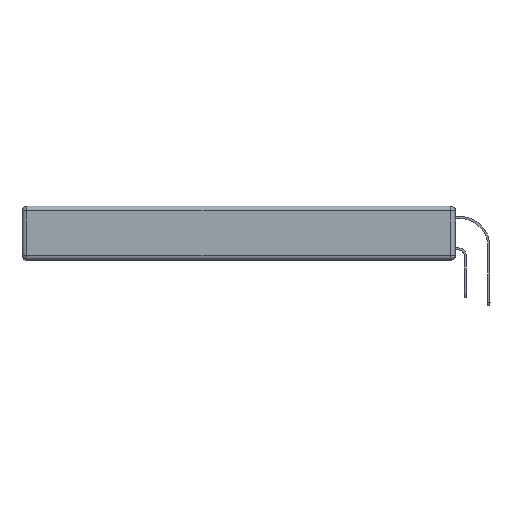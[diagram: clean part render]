
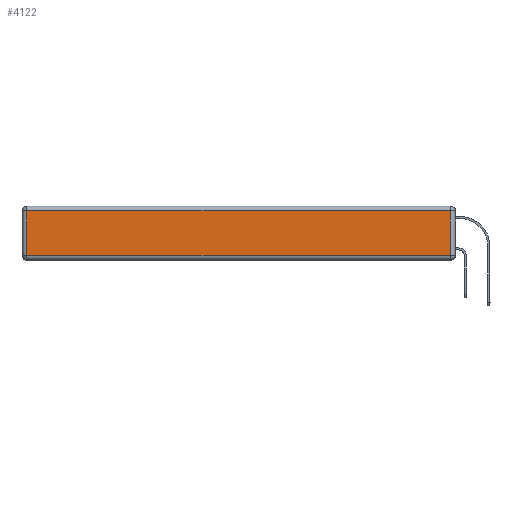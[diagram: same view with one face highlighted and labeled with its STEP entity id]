
A CAD part, left-side view. The second image highlights one B-rep face of the part: STEP entity #4122.
In plain terms, the highlighted planar face has unit normal (-1, 0, 0).
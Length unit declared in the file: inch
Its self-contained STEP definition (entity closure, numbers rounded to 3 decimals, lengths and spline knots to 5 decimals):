
#267 = VECTOR ( 'NONE', #14379, 39.37008 ) ;
#1311 = EDGE_CURVE ( 'NONE', #3050, #4277, #3508, .T. ) ;
#1522 = CARTESIAN_POINT ( 'NONE',  ( 0., 0., -0.343 ) ) ;
#2210 = VECTOR ( 'NONE', #15052, 39.37008 ) ;
#2468 = LINE ( 'NONE', #5930, #2210 ) ;
#3019 = CARTESIAN_POINT ( 'NONE',  ( 0., 2.75, -0.03 ) ) ;
#3050 = VERTEX_POINT ( 'NONE', #3659 ) ;
#3503 = ORIENTED_EDGE ( 'NONE', *, *, #3517, .T. ) ;
#3508 = LINE ( 'NONE', #4664, #5528 ) ;
#3517 = EDGE_CURVE ( 'NONE', #4277, #15799, #14039, .T. ) ;
#3645 = CARTESIAN_POINT ( 'NONE',  ( 0., 2.72, -0.313 ) ) ;
#3659 = CARTESIAN_POINT ( 'NONE',  ( 0., 2.72, -0.03 ) ) ;
#4122 = ADVANCED_FACE ( 'NONE', ( #15659 ), #8351, .T. ) ;
#4127 = VERTEX_POINT ( 'NONE', #14505 ) ;
#4277 = VERTEX_POINT ( 'NONE', #3645 ) ;
#4664 = CARTESIAN_POINT ( 'NONE',  ( 0., 2.72, -0.343 ) ) ;
#5173 = CARTESIAN_POINT ( 'NONE',  ( 0., 0., -0.313 ) ) ;
#5528 = VECTOR ( 'NONE', #8544, 39.37008 ) ;
#5709 = ORIENTED_EDGE ( 'NONE', *, *, #1311, .T. ) ;
#5930 = CARTESIAN_POINT ( 'NONE',  ( 0., 0.03, -0.343 ) ) ;
#6259 = VECTOR ( 'NONE', #12814, 39.37008 ) ;
#6561 = DIRECTION ( 'NONE',  ( 0., 0., 1. ) ) ;
#7049 = CARTESIAN_POINT ( 'NONE',  ( 0., 0.03, -0.313 ) ) ;
#7516 = ORIENTED_EDGE ( 'NONE', *, *, #13819, .T. ) ;
#8351 = PLANE ( 'NONE',  #10190 ) ;
#8544 = DIRECTION ( 'NONE',  ( 0., 0., -1. ) ) ;
#8728 = ORIENTED_EDGE ( 'NONE', *, *, #10016, .T. ) ;
#9124 = DIRECTION ( 'NONE',  ( -1., 0., 0. ) ) ;
#10016 = EDGE_CURVE ( 'NONE', #4127, #3050, #10701, .T. ) ;
#10190 = AXIS2_PLACEMENT_3D ( 'NONE', #1522, #9124, #6561 ) ;
#10701 = LINE ( 'NONE', #3019, #267 ) ;
#12814 = DIRECTION ( 'NONE',  ( 0., -1., 0. ) ) ;
#13467 = EDGE_LOOP ( 'NONE', ( #3503, #7516, #8728, #5709 ) ) ;
#13819 = EDGE_CURVE ( 'NONE', #15799, #4127, #2468, .T. ) ;
#14039 = LINE ( 'NONE', #5173, #6259 ) ;
#14379 = DIRECTION ( 'NONE',  ( 0., 1., 0. ) ) ;
#14505 = CARTESIAN_POINT ( 'NONE',  ( 0., 0.03, -0.03 ) ) ;
#15052 = DIRECTION ( 'NONE',  ( 0., 0., 1. ) ) ;
#15659 = FACE_OUTER_BOUND ( 'NONE', #13467, .T. ) ;
#15799 = VERTEX_POINT ( 'NONE', #7049 ) ;
